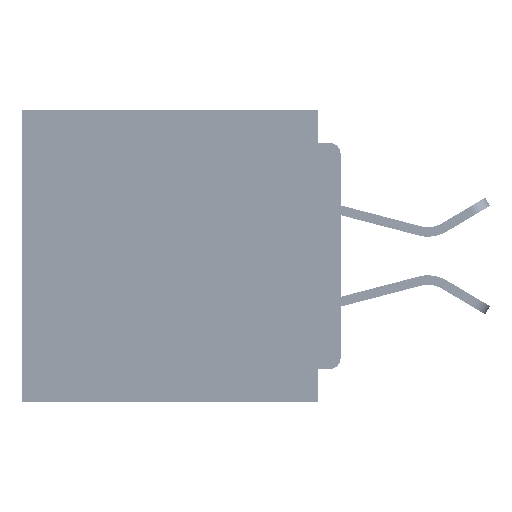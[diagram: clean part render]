
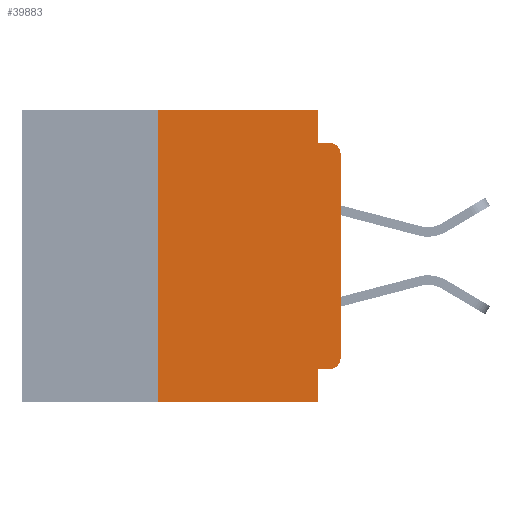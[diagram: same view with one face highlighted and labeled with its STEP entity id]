
A CAD part, left-side view. The second image highlights one B-rep face of the part: STEP entity #39883.
In plain terms, the highlighted planar face has unit normal (-1, 0, 0).
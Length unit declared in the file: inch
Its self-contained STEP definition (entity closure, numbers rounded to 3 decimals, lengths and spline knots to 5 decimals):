
#452 = CARTESIAN_POINT ( 'NONE',  ( 0., 0., -0.045 ) ) ;
#1284 = CARTESIAN_POINT ( 'NONE',  ( 0., 0.015, -0.06 ) ) ;
#1739 = DIRECTION ( 'NONE',  ( 0., 0., -1. ) ) ;
#1901 = VERTEX_POINT ( 'NONE', #36750 ) ;
#2284 = DIRECTION ( 'NONE',  ( 0., 0., -1. ) ) ;
#3669 = EDGE_CURVE ( 'NONE', #11590, #52194, #47023, .T. ) ;
#5142 = DIRECTION ( 'NONE',  ( 0., -1., 0. ) ) ;
#5981 = DIRECTION ( 'NONE',  ( 0., 0., -1. ) ) ;
#6127 = VERTEX_POINT ( 'NONE', #56073 ) ;
#7000 = EDGE_CURVE ( 'NONE', #11590, #12972, #17769, .T. ) ;
#7132 = EDGE_CURVE ( 'NONE', #52194, #6127, #44742, .T. ) ;
#7365 = LINE ( 'NONE', #452, #56916 ) ;
#8023 = CARTESIAN_POINT ( 'NONE',  ( 0., 0.25, -0.4 ) ) ;
#8588 = VECTOR ( 'NONE', #8908, 39.37008 ) ;
#8908 = DIRECTION ( 'NONE',  ( 0., 1., 0. ) ) ;
#9451 = FACE_OUTER_BOUND ( 'NONE', #58580, .T. ) ;
#9753 = ORIENTED_EDGE ( 'NONE', *, *, #38731, .F. ) ;
#10347 = VECTOR ( 'NONE', #2284, 39.37008 ) ;
#11413 = VECTOR ( 'NONE', #53522, 39.37008 ) ;
#11485 = CARTESIAN_POINT ( 'NONE',  ( 0., 0.031, 0. ) ) ;
#11590 = VERTEX_POINT ( 'NONE', #8023 ) ;
#11961 = LINE ( 'NONE', #45190, #60020 ) ;
#12972 = VERTEX_POINT ( 'NONE', #32632 ) ;
#17281 = DIRECTION ( 'NONE',  ( 0., -1., 0. ) ) ;
#17761 = ORIENTED_EDGE ( 'NONE', *, *, #58774, .T. ) ;
#17769 = LINE ( 'NONE', #20788, #53444 ) ;
#19278 = ORIENTED_EDGE ( 'NONE', *, *, #42180, .F. ) ;
#19365 = EDGE_CURVE ( 'NONE', #50293, #39172, #37716, .T. ) ;
#20788 = CARTESIAN_POINT ( 'NONE',  ( 0., 0.437, -0.4 ) ) ;
#22107 = ORIENTED_EDGE ( 'NONE', *, *, #26654, .F. ) ;
#23445 = DIRECTION ( 'NONE',  ( -1., 0., 0. ) ) ;
#24259 = LINE ( 'NONE', #11485, #10347 ) ;
#24324 = CARTESIAN_POINT ( 'NONE',  ( 0., 0., -0.06 ) ) ;
#25506 = DIRECTION ( 'NONE',  ( 0., -1., 0. ) ) ;
#25517 = AXIS2_PLACEMENT_3D ( 'NONE', #1284, #33992, #5981 ) ;
#26654 = EDGE_CURVE ( 'NONE', #27068, #12972, #11961, .T. ) ;
#27068 = VERTEX_POINT ( 'NONE', #47979 ) ;
#27926 = CARTESIAN_POINT ( 'NONE',  ( 0., 0.25, -0.4 ) ) ;
#28492 = CARTESIAN_POINT ( 'NONE',  ( 0., 0.031, -0.045 ) ) ;
#29779 = DIRECTION ( 'NONE',  ( 1., 0., 0. ) ) ;
#29780 = ORIENTED_EDGE ( 'NONE', *, *, #7132, .F. ) ;
#30986 = CARTESIAN_POINT ( 'NONE',  ( 0., 0.015, -0.355 ) ) ;
#32397 = VECTOR ( 'NONE', #17281, 39.37008 ) ;
#32632 = CARTESIAN_POINT ( 'NONE',  ( 0., 0.031, -0.4 ) ) ;
#33487 = LINE ( 'NONE', #36903, #8588 ) ;
#33630 = ORIENTED_EDGE ( 'NONE', *, *, #39626, .T. ) ;
#33992 = DIRECTION ( 'NONE',  ( -1., 0., 0. ) ) ;
#34402 = ORIENTED_EDGE ( 'NONE', *, *, #19365, .T. ) ;
#34679 = VECTOR ( 'NONE', #55736, 39.37008 ) ;
#35897 = ORIENTED_EDGE ( 'NONE', *, *, #47158, .F. ) ;
#36750 = CARTESIAN_POINT ( 'NONE',  ( 0., 0.015, -0.045 ) ) ;
#36903 = CARTESIAN_POINT ( 'NONE',  ( 0., 0., -0.355 ) ) ;
#37716 = LINE ( 'NONE', #48882, #11413 ) ;
#38731 = EDGE_CURVE ( 'NONE', #6127, #51380, #24259, .T. ) ;
#39172 = VERTEX_POINT ( 'NONE', #24324 ) ;
#39626 = EDGE_CURVE ( 'NONE', #40052, #50293, #45990, .T. ) ;
#39883 = ADVANCED_FACE ( 'NONE', ( #9451 ), #57571, .F. ) ;
#40052 = VERTEX_POINT ( 'NONE', #30986 ) ;
#40551 = ORIENTED_EDGE ( 'NONE', *, *, #7000, .T. ) ;
#41506 = CIRCLE ( 'NONE', #25517, 0.015 ) ;
#42180 = EDGE_CURVE ( 'NONE', #40052, #27068, #33487, .T. ) ;
#44742 = LINE ( 'NONE', #45220, #32397 ) ;
#45063 = ORIENTED_EDGE ( 'NONE', *, *, #3669, .F. ) ;
#45190 = CARTESIAN_POINT ( 'NONE',  ( 0., 0.031, -0.4 ) ) ;
#45220 = CARTESIAN_POINT ( 'NONE',  ( 0., 0.437, 0. ) ) ;
#45990 = CIRCLE ( 'NONE', #58836, 0.015 ) ;
#47023 = LINE ( 'NONE', #27926, #34679 ) ;
#47100 = CARTESIAN_POINT ( 'NONE',  ( 0., 0., -0.34 ) ) ;
#47158 = EDGE_CURVE ( 'NONE', #51380, #1901, #7365, .T. ) ;
#47268 = CARTESIAN_POINT ( 'NONE',  ( 0., 0.25, 0. ) ) ;
#47979 = CARTESIAN_POINT ( 'NONE',  ( 0., 0.031, -0.355 ) ) ;
#48252 = CARTESIAN_POINT ( 'NONE',  ( 0., 0.437, 0. ) ) ;
#48882 = CARTESIAN_POINT ( 'NONE',  ( 0., 0., 0. ) ) ;
#50293 = VERTEX_POINT ( 'NONE', #47100 ) ;
#51305 = CARTESIAN_POINT ( 'NONE',  ( 0., 0.015, -0.34 ) ) ;
#51380 = VERTEX_POINT ( 'NONE', #28492 ) ;
#52194 = VERTEX_POINT ( 'NONE', #47268 ) ;
#53444 = VECTOR ( 'NONE', #25506, 39.37008 ) ;
#53522 = DIRECTION ( 'NONE',  ( 0., 0., 1. ) ) ;
#54575 = AXIS2_PLACEMENT_3D ( 'NONE', #48252, #29779, #1739 ) ;
#55736 = DIRECTION ( 'NONE',  ( 0., 0., 1. ) ) ;
#55958 = DIRECTION ( 'NONE',  ( 0., 0., -1. ) ) ;
#56073 = CARTESIAN_POINT ( 'NONE',  ( 0., 0.031, 0. ) ) ;
#56916 = VECTOR ( 'NONE', #5142, 39.37008 ) ;
#57571 = PLANE ( 'NONE',  #54575 ) ;
#58580 = EDGE_LOOP ( 'NONE', ( #34402, #17761, #35897, #9753, #29780, #45063, #40551, #22107, #19278, #33630 ) ) ;
#58774 = EDGE_CURVE ( 'NONE', #39172, #1901, #41506, .T. ) ;
#58836 = AXIS2_PLACEMENT_3D ( 'NONE', #51305, #23445, #55958 ) ;
#59158 = DIRECTION ( 'NONE',  ( 0., 0., -1. ) ) ;
#60020 = VECTOR ( 'NONE', #59158, 39.37008 ) ;
